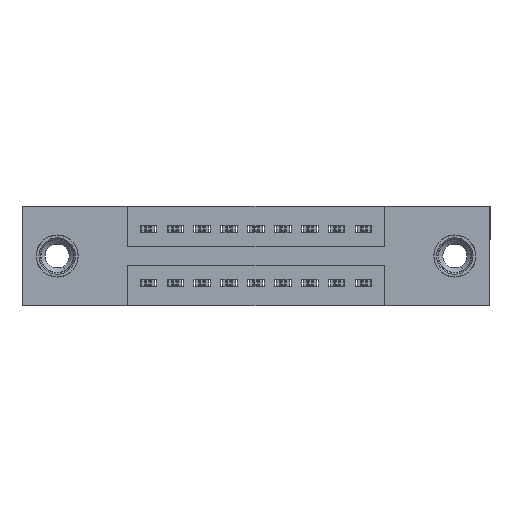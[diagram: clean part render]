
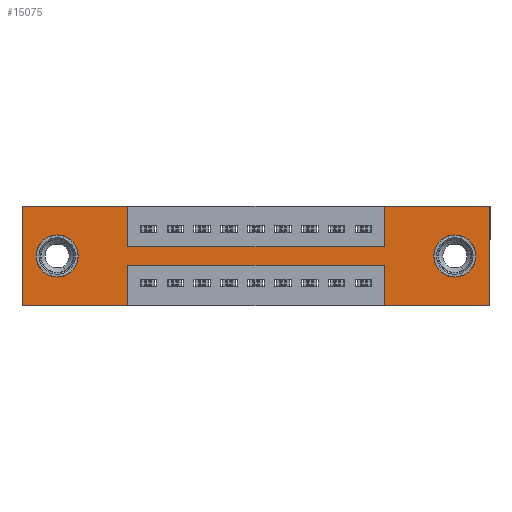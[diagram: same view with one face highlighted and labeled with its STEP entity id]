
A CAD part, front view. The second image highlights one B-rep face of the part: STEP entity #15075.
In plain terms, the highlighted planar face has unit normal (0, -1, 0).
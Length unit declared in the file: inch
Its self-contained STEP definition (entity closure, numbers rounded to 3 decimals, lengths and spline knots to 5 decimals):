
#107 = ORIENTED_EDGE ( 'NONE', *, *, #12367, .T. ) ;
#503 = CARTESIAN_POINT ( 'NONE',  ( 0.13, 0., -0.185 ) ) ;
#567 = CARTESIAN_POINT ( 'NONE',  ( 0., 0., -0.37 ) ) ;
#609 = CARTESIAN_POINT ( 'NONE',  ( 0., 0., 0. ) ) ;
#705 = LINE ( 'NONE', #13201, #4787 ) ;
#746 = ORIENTED_EDGE ( 'NONE', *, *, #1278, .F. ) ;
#775 = VERTEX_POINT ( 'NONE', #5000 ) ;
#826 = DIRECTION ( 'NONE',  ( 0., 0., 1. ) ) ;
#831 = ORIENTED_EDGE ( 'NONE', *, *, #13731, .F. ) ;
#836 = VERTEX_POINT ( 'NONE', #3595 ) ;
#1068 = VECTOR ( 'NONE', #6340, 39.37008 ) ;
#1278 = EDGE_CURVE ( 'NONE', #5326, #11371, #3989, .T. ) ;
#1340 = EDGE_CURVE ( 'NONE', #4072, #10090, #12580, .T. ) ;
#1343 = VECTOR ( 'NONE', #14430, 39.37008 ) ;
#1394 = CIRCLE ( 'NONE', #3777, 0.078 ) ;
#1452 = CARTESIAN_POINT ( 'NONE',  ( 0.3925, 0., -0.37 ) ) ;
#1461 = DIRECTION ( 'NONE',  ( 0., 0., -1. ) ) ;
#1602 = VECTOR ( 'NONE', #14532, 39.37008 ) ;
#1710 = PLANE ( 'NONE',  #3843 ) ;
#1737 = LINE ( 'NONE', #8143, #10939 ) ;
#1782 = DIRECTION ( 'NONE',  ( 0., 0., -1. ) ) ;
#1897 = CARTESIAN_POINT ( 'NONE',  ( 0.13, 0., -0.185 ) ) ;
#1965 = LINE ( 'NONE', #9831, #12531 ) ;
#2068 = DIRECTION ( 'NONE',  ( 0., 1., 0. ) ) ;
#2105 = CIRCLE ( 'NONE', #10580, 0.078 ) ;
#2279 = VERTEX_POINT ( 'NONE', #9667 ) ;
#2465 = AXIS2_PLACEMENT_3D ( 'NONE', #3697, #8767, #11015 ) ;
#2529 = ORIENTED_EDGE ( 'NONE', *, *, #12543, .F. ) ;
#2702 = FACE_BOUND ( 'NONE', #8643, .T. ) ;
#2965 = ORIENTED_EDGE ( 'NONE', *, *, #9877, .F. ) ;
#2993 = ORIENTED_EDGE ( 'NONE', *, *, #10430, .F. ) ;
#3065 = CARTESIAN_POINT ( 'NONE',  ( 1.3425, 0., -0.22 ) ) ;
#3209 = VECTOR ( 'NONE', #6744, 39.37008 ) ;
#3595 = CARTESIAN_POINT ( 'NONE',  ( 1.605, 0., -0.263 ) ) ;
#3650 = CARTESIAN_POINT ( 'NONE',  ( 0.3925, 0., -0.37 ) ) ;
#3697 = CARTESIAN_POINT ( 'NONE',  ( 1.605, 0., -0.185 ) ) ;
#3777 = AXIS2_PLACEMENT_3D ( 'NONE', #503, #4402, #826 ) ;
#3805 = CARTESIAN_POINT ( 'NONE',  ( 1.735, 0., -0.37 ) ) ;
#3843 = AXIS2_PLACEMENT_3D ( 'NONE', #4044, #7773, #1461 ) ;
#3901 = EDGE_CURVE ( 'NONE', #11371, #6669, #5996, .T. ) ;
#3989 = LINE ( 'NONE', #9044, #14415 ) ;
#4001 = VERTEX_POINT ( 'NONE', #10358 ) ;
#4044 = CARTESIAN_POINT ( 'NONE',  ( 0., 0., -0.37 ) ) ;
#4072 = VERTEX_POINT ( 'NONE', #10599 ) ;
#4088 = VERTEX_POINT ( 'NONE', #3065 ) ;
#4402 = DIRECTION ( 'NONE',  ( 0., 1., 0. ) ) ;
#4418 = EDGE_CURVE ( 'NONE', #6700, #4745, #11962, .T. ) ;
#4663 = ORIENTED_EDGE ( 'NONE', *, *, #9767, .F. ) ;
#4711 = CARTESIAN_POINT ( 'NONE',  ( 0., 0., -0.37 ) ) ;
#4745 = VERTEX_POINT ( 'NONE', #14083 ) ;
#4787 = VECTOR ( 'NONE', #1782, 39.37008 ) ;
#5000 = CARTESIAN_POINT ( 'NONE',  ( 0.3925, 0., -0.15 ) ) ;
#5326 = VERTEX_POINT ( 'NONE', #13728 ) ;
#5599 = EDGE_CURVE ( 'NONE', #4745, #2279, #1737, .T. ) ;
#5917 = EDGE_LOOP ( 'NONE', ( #13191, #107 ) ) ;
#5996 = LINE ( 'NONE', #14890, #10105 ) ;
#6340 = DIRECTION ( 'NONE',  ( 1., 0., 0. ) ) ;
#6669 = VERTEX_POINT ( 'NONE', #15145 ) ;
#6700 = VERTEX_POINT ( 'NONE', #567 ) ;
#6744 = DIRECTION ( 'NONE',  ( 1., 0., 0. ) ) ;
#6794 = DIRECTION ( 'NONE',  ( 1., 0., 0. ) ) ;
#6941 = EDGE_CURVE ( 'NONE', #836, #4001, #2105, .T. ) ;
#7127 = LINE ( 'NONE', #15778, #1602 ) ;
#7408 = DIRECTION ( 'NONE',  ( 0., 0., -1. ) ) ;
#7511 = CIRCLE ( 'NONE', #2465, 0.078 ) ;
#7609 = VERTEX_POINT ( 'NONE', #13667 ) ;
#7627 = EDGE_CURVE ( 'NONE', #15791, #8594, #11274, .T. ) ;
#7664 = LINE ( 'NONE', #7920, #3209 ) ;
#7773 = DIRECTION ( 'NONE',  ( 0., -1., 0. ) ) ;
#7920 = CARTESIAN_POINT ( 'NONE',  ( 0.3925, 0., -0.15 ) ) ;
#8052 = CARTESIAN_POINT ( 'NONE',  ( 0.3925, 0., -0.22 ) ) ;
#8143 = CARTESIAN_POINT ( 'NONE',  ( 0., 0., 0. ) ) ;
#8154 = DIRECTION ( 'NONE',  ( 0., 0., 1. ) ) ;
#8594 = VERTEX_POINT ( 'NONE', #1452 ) ;
#8602 = EDGE_CURVE ( 'NONE', #16077, #5326, #8992, .T. ) ;
#8643 = EDGE_LOOP ( 'NONE', ( #9218, #15085 ) ) ;
#8767 = DIRECTION ( 'NONE',  ( 0., 1., 0. ) ) ;
#8992 = LINE ( 'NONE', #14109, #1068 ) ;
#9014 = CARTESIAN_POINT ( 'NONE',  ( 1.605, 0., -0.185 ) ) ;
#9044 = CARTESIAN_POINT ( 'NONE',  ( 1.735, 0., 0. ) ) ;
#9218 = ORIENTED_EDGE ( 'NONE', *, *, #12687, .T. ) ;
#9259 = FACE_BOUND ( 'NONE', #5917, .T. ) ;
#9453 = LINE ( 'NONE', #8052, #14596 ) ;
#9508 = ORIENTED_EDGE ( 'NONE', *, *, #10237, .F. ) ;
#9667 = CARTESIAN_POINT ( 'NONE',  ( 0.3925, 0., 0. ) ) ;
#9767 = EDGE_CURVE ( 'NONE', #8594, #6700, #13301, .T. ) ;
#9831 = CARTESIAN_POINT ( 'NONE',  ( 1.3425, 0., 0. ) ) ;
#9877 = EDGE_CURVE ( 'NONE', #6669, #4088, #7127, .T. ) ;
#9942 = DIRECTION ( 'NONE',  ( -1., 0., 0. ) ) ;
#10048 = VECTOR ( 'NONE', #7408, 39.37008 ) ;
#10090 = VERTEX_POINT ( 'NONE', #10497 ) ;
#10105 = VECTOR ( 'NONE', #9942, 39.37008 ) ;
#10237 = EDGE_CURVE ( 'NONE', #2279, #775, #705, .T. ) ;
#10358 = CARTESIAN_POINT ( 'NONE',  ( 1.605, 0., -0.107 ) ) ;
#10430 = EDGE_CURVE ( 'NONE', #775, #7609, #7664, .T. ) ;
#10497 = CARTESIAN_POINT ( 'NONE',  ( 0.13, 0., -0.263 ) ) ;
#10580 = AXIS2_PLACEMENT_3D ( 'NONE', #9014, #12732, #15279 ) ;
#10599 = CARTESIAN_POINT ( 'NONE',  ( 0.13, 0., -0.107 ) ) ;
#10820 = ORIENTED_EDGE ( 'NONE', *, *, #4418, .F. ) ;
#10918 = DIRECTION ( 'NONE',  ( -1., 0., 0. ) ) ;
#10939 = VECTOR ( 'NONE', #6794, 39.37008 ) ;
#11015 = DIRECTION ( 'NONE',  ( 0., 0., -1. ) ) ;
#11274 = LINE ( 'NONE', #3650, #10048 ) ;
#11371 = VERTEX_POINT ( 'NONE', #3805 ) ;
#11395 = ORIENTED_EDGE ( 'NONE', *, *, #5599, .F. ) ;
#11612 = ORIENTED_EDGE ( 'NONE', *, *, #7627, .F. ) ;
#11962 = LINE ( 'NONE', #609, #1343 ) ;
#12367 = EDGE_CURVE ( 'NONE', #10090, #4072, #1394, .T. ) ;
#12531 = VECTOR ( 'NONE', #13949, 39.37008 ) ;
#12543 = EDGE_CURVE ( 'NONE', #4088, #15791, #9453, .T. ) ;
#12580 = CIRCLE ( 'NONE', #12855, 0.078 ) ;
#12687 = EDGE_CURVE ( 'NONE', #4001, #836, #7511, .T. ) ;
#12732 = DIRECTION ( 'NONE',  ( 0., 1., 0. ) ) ;
#12836 = ORIENTED_EDGE ( 'NONE', *, *, #8602, .F. ) ;
#12855 = AXIS2_PLACEMENT_3D ( 'NONE', #1897, #2068, #8154 ) ;
#12996 = CARTESIAN_POINT ( 'NONE',  ( 0.3925, 0., -0.22 ) ) ;
#13191 = ORIENTED_EDGE ( 'NONE', *, *, #1340, .T. ) ;
#13201 = CARTESIAN_POINT ( 'NONE',  ( 0.3925, 0., 0. ) ) ;
#13301 = LINE ( 'NONE', #4711, #15593 ) ;
#13309 = DIRECTION ( 'NONE',  ( -1., 0., 0. ) ) ;
#13667 = CARTESIAN_POINT ( 'NONE',  ( 1.3425, 0., -0.15 ) ) ;
#13728 = CARTESIAN_POINT ( 'NONE',  ( 1.735, 0., 0. ) ) ;
#13731 = EDGE_CURVE ( 'NONE', #7609, #16077, #1965, .T. ) ;
#13949 = DIRECTION ( 'NONE',  ( 0., 0., 1. ) ) ;
#14032 = CARTESIAN_POINT ( 'NONE',  ( 1.3425, 0., 0. ) ) ;
#14065 = DIRECTION ( 'NONE',  ( 0., 0., -1. ) ) ;
#14083 = CARTESIAN_POINT ( 'NONE',  ( 0., 0., 0. ) ) ;
#14109 = CARTESIAN_POINT ( 'NONE',  ( 0., 0., 0. ) ) ;
#14269 = FACE_OUTER_BOUND ( 'NONE', #15213, .T. ) ;
#14415 = VECTOR ( 'NONE', #14065, 39.37008 ) ;
#14430 = DIRECTION ( 'NONE',  ( 0., 0., 1. ) ) ;
#14532 = DIRECTION ( 'NONE',  ( 0., 0., 1. ) ) ;
#14596 = VECTOR ( 'NONE', #13309, 39.37008 ) ;
#14890 = CARTESIAN_POINT ( 'NONE',  ( 0., 0., -0.37 ) ) ;
#15075 = ADVANCED_FACE ( 'NONE', ( #2702, #9259, #14269 ), #1710, .T. ) ;
#15085 = ORIENTED_EDGE ( 'NONE', *, *, #6941, .T. ) ;
#15145 = CARTESIAN_POINT ( 'NONE',  ( 1.3425, 0., -0.37 ) ) ;
#15213 = EDGE_LOOP ( 'NONE', ( #11612, #2529, #2965, #16073, #746, #12836, #831, #2993, #9508, #11395, #10820, #4663 ) ) ;
#15279 = DIRECTION ( 'NONE',  ( 0., 0., -1. ) ) ;
#15593 = VECTOR ( 'NONE', #10918, 39.37008 ) ;
#15778 = CARTESIAN_POINT ( 'NONE',  ( 1.3425, 0., -0.37 ) ) ;
#15791 = VERTEX_POINT ( 'NONE', #12996 ) ;
#16073 = ORIENTED_EDGE ( 'NONE', *, *, #3901, .F. ) ;
#16077 = VERTEX_POINT ( 'NONE', #14032 ) ;
